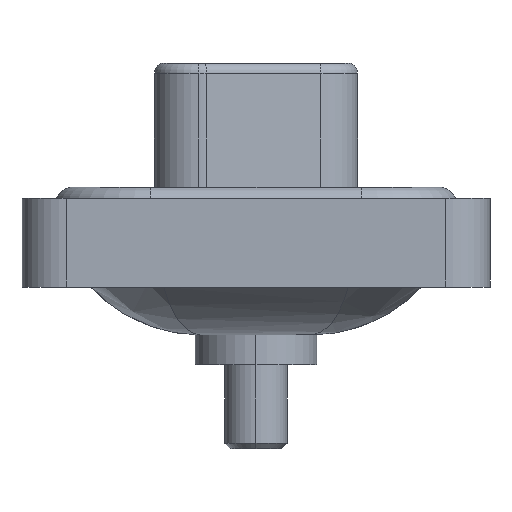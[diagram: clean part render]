
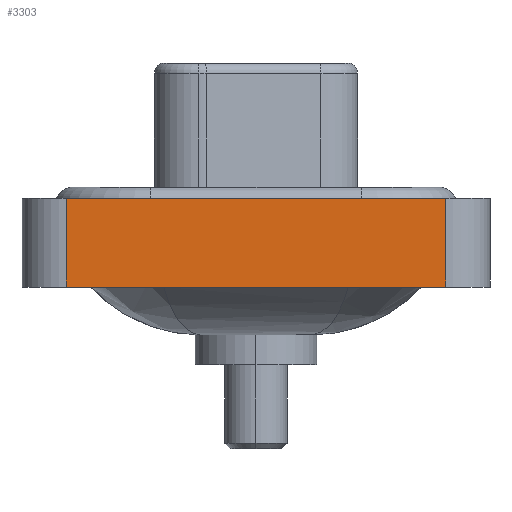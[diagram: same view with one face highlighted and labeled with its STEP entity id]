
A CAD part, left-side view. The second image highlights one B-rep face of the part: STEP entity #3303.
In plain terms, the highlighted planar face has unit normal (-1, 0, 0).
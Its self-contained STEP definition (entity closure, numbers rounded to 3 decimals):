
#54 = ORIENTED_EDGE ( 'NONE', *, *, #6628, .F. ) ;
#143 = VERTEX_POINT ( 'NONE', #9147 ) ;
#242 = ORIENTED_EDGE ( 'NONE', *, *, #464, .T. ) ;
#464 = EDGE_CURVE ( 'NONE', #1668, #5328, #4073, .T. ) ;
#915 = CARTESIAN_POINT ( 'NONE',  ( -7.25, -8.55, -3.6 ) ) ;
#1668 = VERTEX_POINT ( 'NONE', #8160 ) ;
#2328 = DIRECTION ( 'NONE',  ( -1., 0., 0. ) ) ;
#3269 = VECTOR ( 'NONE', #12079, 1000. ) ;
#3303 = ADVANCED_FACE ( 'NONE', ( #5971 ), #3481, .T. ) ;
#3377 = CARTESIAN_POINT ( 'NONE',  ( -7.25, 8.55, -3.6 ) ) ;
#3481 = PLANE ( 'NONE',  #12541 ) ;
#4007 = VECTOR ( 'NONE', #7490, 1000. ) ;
#4073 = LINE ( 'NONE', #11211, #4007 ) ;
#4101 = VERTEX_POINT ( 'NONE', #5754 ) ;
#4331 = EDGE_LOOP ( 'NONE', ( #242, #7317, #54, #14688 ) ) ;
#5328 = VERTEX_POINT ( 'NONE', #14280 ) ;
#5754 = CARTESIAN_POINT ( 'NONE',  ( -7.25, 8.55, -3.6 ) ) ;
#5940 = LINE ( 'NONE', #3377, #13466 ) ;
#5971 = FACE_OUTER_BOUND ( 'NONE', #4331, .T. ) ;
#6390 = EDGE_CURVE ( 'NONE', #143, #5328, #11075, .T. ) ;
#6628 = EDGE_CURVE ( 'NONE', #4101, #143, #5940, .T. ) ;
#7052 = DIRECTION ( 'NONE',  ( 0., 0., 1. ) ) ;
#7317 = ORIENTED_EDGE ( 'NONE', *, *, #6390, .F. ) ;
#7490 = DIRECTION ( 'NONE',  ( 0., 0., 1. ) ) ;
#8160 = CARTESIAN_POINT ( 'NONE',  ( -7.25, -8.55, -3.6 ) ) ;
#8190 = DIRECTION ( 'NONE',  ( 0., 0., 1. ) ) ;
#9147 = CARTESIAN_POINT ( 'NONE',  ( -7.25, 8.55, 0.4 ) ) ;
#11075 = LINE ( 'NONE', #14387, #3269 ) ;
#11211 = CARTESIAN_POINT ( 'NONE',  ( -7.25, -8.55, -3.6 ) ) ;
#11437 = LINE ( 'NONE', #915, #14662 ) ;
#11737 = EDGE_CURVE ( 'NONE', #4101, #1668, #11437, .T. ) ;
#12079 = DIRECTION ( 'NONE',  ( 0., -1., 0. ) ) ;
#12541 = AXIS2_PLACEMENT_3D ( 'NONE', #12936, #2328, #7052 ) ;
#12936 = CARTESIAN_POINT ( 'NONE',  ( -7.25, -8.55, -3.6 ) ) ;
#13466 = VECTOR ( 'NONE', #8190, 1000. ) ;
#14054 = DIRECTION ( 'NONE',  ( 0., -1., 0. ) ) ;
#14280 = CARTESIAN_POINT ( 'NONE',  ( -7.25, -8.55, 0.4 ) ) ;
#14387 = CARTESIAN_POINT ( 'NONE',  ( -7.25, -8.55, 0.4 ) ) ;
#14662 = VECTOR ( 'NONE', #14054, 1000. ) ;
#14688 = ORIENTED_EDGE ( 'NONE', *, *, #11737, .T. ) ;
